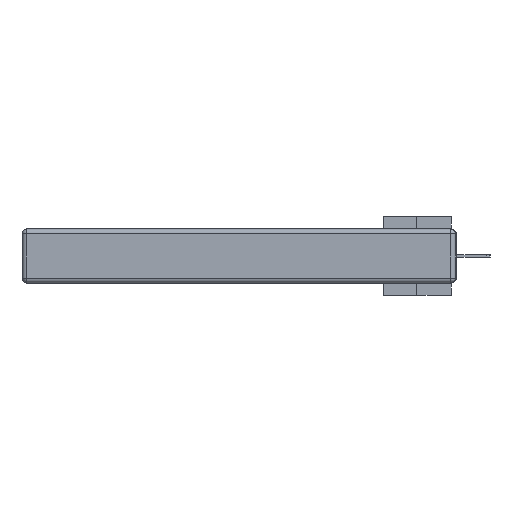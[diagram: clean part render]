
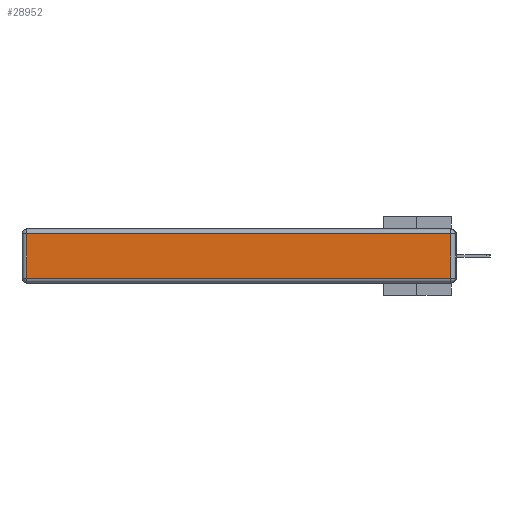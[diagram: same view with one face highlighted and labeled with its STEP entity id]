
A CAD part, left-side view. The second image highlights one B-rep face of the part: STEP entity #28952.
In plain terms, the highlighted planar face has unit normal (-1, 0, 0).
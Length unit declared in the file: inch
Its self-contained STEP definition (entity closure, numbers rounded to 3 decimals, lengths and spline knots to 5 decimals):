
#271 = EDGE_CURVE ( 'NONE', #24835, #33487, #18705, .T. ) ;
#516 = VECTOR ( 'NONE', #19816, 39.37008 ) ;
#1382 = VERTEX_POINT ( 'NONE', #35117 ) ;
#1605 = EDGE_CURVE ( 'NONE', #1382, #32871, #35954, .T. ) ;
#1862 = PLANE ( 'NONE',  #20198 ) ;
#3084 = ORIENTED_EDGE ( 'NONE', *, *, #33233, .T. ) ;
#5036 = DIRECTION ( 'NONE',  ( -1., 0., 0. ) ) ;
#9846 = LINE ( 'NONE', #13626, #516 ) ;
#10409 = DIRECTION ( 'NONE',  ( 0., 1., 0. ) ) ;
#10489 = CARTESIAN_POINT ( 'NONE',  ( 0., 2.75, -0.03 ) ) ;
#13626 = CARTESIAN_POINT ( 'NONE',  ( 0., 2.72, -0.343 ) ) ;
#14361 = CARTESIAN_POINT ( 'NONE',  ( 0., 0., -0.343 ) ) ;
#18554 = DIRECTION ( 'NONE',  ( 0., 0., 1. ) ) ;
#18705 = LINE ( 'NONE', #10489, #25073 ) ;
#18828 = ORIENTED_EDGE ( 'NONE', *, *, #1605, .T. ) ;
#19566 = VECTOR ( 'NONE', #27112, 39.37008 ) ;
#19816 = DIRECTION ( 'NONE',  ( 0., 0., -1. ) ) ;
#20198 = AXIS2_PLACEMENT_3D ( 'NONE', #14361, #5036, #26970 ) ;
#20802 = CARTESIAN_POINT ( 'NONE',  ( 0., 0.03, -0.313 ) ) ;
#21329 = CARTESIAN_POINT ( 'NONE',  ( 0., 0., -0.313 ) ) ;
#22790 = ORIENTED_EDGE ( 'NONE', *, *, #271, .T. ) ;
#23151 = EDGE_LOOP ( 'NONE', ( #18828, #33867, #22790, #3084 ) ) ;
#24309 = CARTESIAN_POINT ( 'NONE',  ( 0., 2.72, -0.03 ) ) ;
#24835 = VERTEX_POINT ( 'NONE', #24954 ) ;
#24954 = CARTESIAN_POINT ( 'NONE',  ( 0., 0.03, -0.03 ) ) ;
#25073 = VECTOR ( 'NONE', #10409, 39.37008 ) ;
#26970 = DIRECTION ( 'NONE',  ( 0., 0., 1. ) ) ;
#27112 = DIRECTION ( 'NONE',  ( 0., -1., 0. ) ) ;
#28952 = ADVANCED_FACE ( 'NONE', ( #38295 ), #1862, .T. ) ;
#29078 = VECTOR ( 'NONE', #18554, 39.37008 ) ;
#30889 = CARTESIAN_POINT ( 'NONE',  ( 0., 0.03, -0.343 ) ) ;
#31725 = EDGE_CURVE ( 'NONE', #32871, #24835, #37169, .T. ) ;
#32871 = VERTEX_POINT ( 'NONE', #20802 ) ;
#33233 = EDGE_CURVE ( 'NONE', #33487, #1382, #9846, .T. ) ;
#33487 = VERTEX_POINT ( 'NONE', #24309 ) ;
#33867 = ORIENTED_EDGE ( 'NONE', *, *, #31725, .T. ) ;
#35117 = CARTESIAN_POINT ( 'NONE',  ( 0., 2.72, -0.313 ) ) ;
#35954 = LINE ( 'NONE', #21329, #19566 ) ;
#37169 = LINE ( 'NONE', #30889, #29078 ) ;
#38295 = FACE_OUTER_BOUND ( 'NONE', #23151, .T. ) ;
